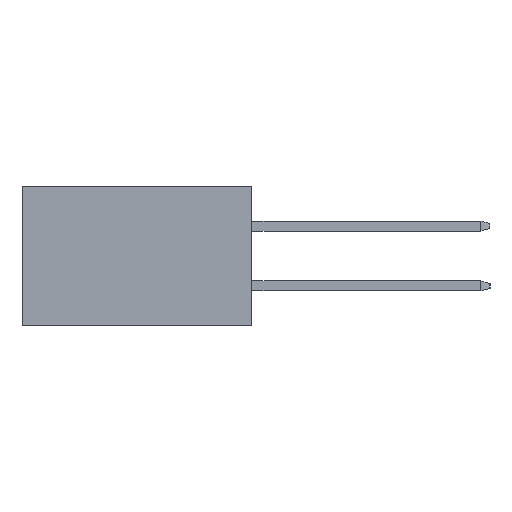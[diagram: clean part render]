
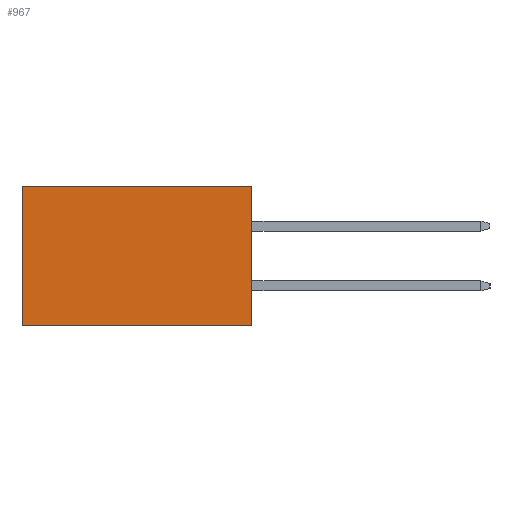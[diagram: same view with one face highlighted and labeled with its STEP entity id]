
A CAD part, left-side view. The second image highlights one B-rep face of the part: STEP entity #967.
In plain terms, the highlighted planar face has unit normal (-1, 0, 0).
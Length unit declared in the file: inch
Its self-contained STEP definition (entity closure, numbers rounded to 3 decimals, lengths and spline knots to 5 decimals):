
#591 = CARTESIAN_POINT ( 'NONE',  ( 0.3205, 0., -0.437 ) ) ;
#967 = ADVANCED_FACE ( 'NONE', ( #7211 ), #16495, .F. ) ;
#1712 = CARTESIAN_POINT ( 'NONE',  ( 0.3205, 0., -0.437 ) ) ;
#1901 = CARTESIAN_POINT ( 'NONE',  ( 0.3205, 0.72, -0.437 ) ) ;
#3026 = ORIENTED_EDGE ( 'NONE', *, *, #17059, .F. ) ;
#3199 = DIRECTION ( 'NONE',  ( 0., 1., 0. ) ) ;
#3691 = DIRECTION ( 'NONE',  ( 0., 0., -1. ) ) ;
#4999 = CARTESIAN_POINT ( 'NONE',  ( 0.3205, 0.72, 0. ) ) ;
#5377 = CARTESIAN_POINT ( 'NONE',  ( 0.3205, 0., 0. ) ) ;
#6639 = CARTESIAN_POINT ( 'NONE',  ( 0.3205, 0., -0.437 ) ) ;
#6795 = DIRECTION ( 'NONE',  ( 0., 0., -1. ) ) ;
#6823 = VECTOR ( 'NONE', #6890, 39.37008 ) ;
#6890 = DIRECTION ( 'NONE',  ( 0., 1., 0. ) ) ;
#7211 = FACE_OUTER_BOUND ( 'NONE', #13134, .T. ) ;
#7777 = VECTOR ( 'NONE', #3199, 39.37008 ) ;
#8187 = LINE ( 'NONE', #17374, #10008 ) ;
#9006 = VERTEX_POINT ( 'NONE', #4999 ) ;
#9055 = ORIENTED_EDGE ( 'NONE', *, *, #14446, .T. ) ;
#10008 = VECTOR ( 'NONE', #3691, 39.37008 ) ;
#10187 = DIRECTION ( 'NONE',  ( 0., 0., -1. ) ) ;
#11603 = DIRECTION ( 'NONE',  ( 1., 0., 0. ) ) ;
#12670 = AXIS2_PLACEMENT_3D ( 'NONE', #6639, #11603, #10187 ) ;
#13134 = EDGE_LOOP ( 'NONE', ( #9055, #18991, #3026, #19651 ) ) ;
#13264 = LINE ( 'NONE', #5377, #6823 ) ;
#13866 = VECTOR ( 'NONE', #6795, 39.37008 ) ;
#14446 = EDGE_CURVE ( 'NONE', #9006, #18435, #8187, .T. ) ;
#14542 = EDGE_CURVE ( 'NONE', #17581, #18435, #18497, .T. ) ;
#16126 = EDGE_CURVE ( 'NONE', #17388, #9006, #13264, .T. ) ;
#16495 = PLANE ( 'NONE',  #12670 ) ;
#17059 = EDGE_CURVE ( 'NONE', #17388, #17581, #18889, .T. ) ;
#17374 = CARTESIAN_POINT ( 'NONE',  ( 0.3205, 0.72, -0.437 ) ) ;
#17388 = VERTEX_POINT ( 'NONE', #18378 ) ;
#17581 = VERTEX_POINT ( 'NONE', #18469 ) ;
#18378 = CARTESIAN_POINT ( 'NONE',  ( 0.3205, 0., 0. ) ) ;
#18435 = VERTEX_POINT ( 'NONE', #1901 ) ;
#18469 = CARTESIAN_POINT ( 'NONE',  ( 0.3205, 0., -0.437 ) ) ;
#18497 = LINE ( 'NONE', #1712, #7777 ) ;
#18889 = LINE ( 'NONE', #591, #13866 ) ;
#18991 = ORIENTED_EDGE ( 'NONE', *, *, #14542, .F. ) ;
#19651 = ORIENTED_EDGE ( 'NONE', *, *, #16126, .T. ) ;
